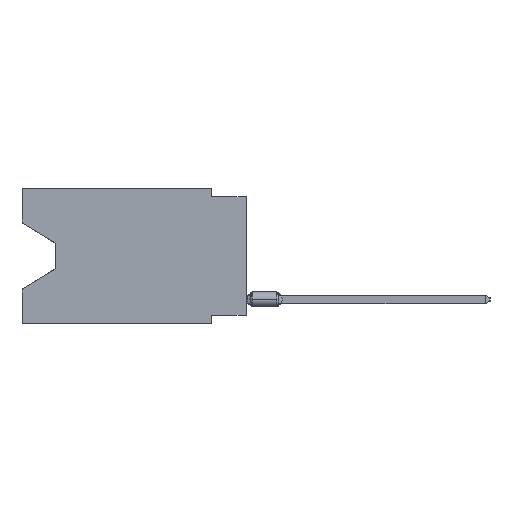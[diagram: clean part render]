
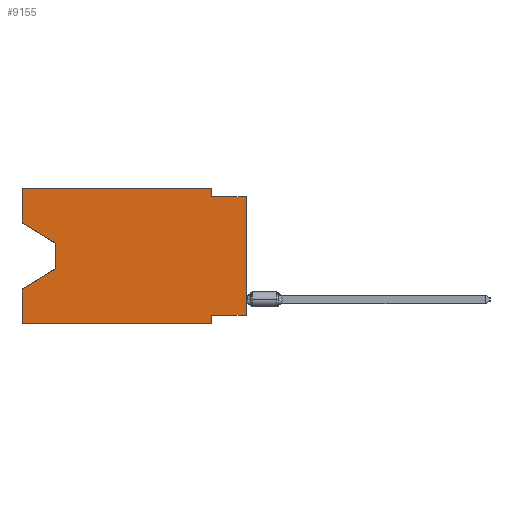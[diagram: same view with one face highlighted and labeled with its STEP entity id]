
A CAD part, left-side view. The second image highlights one B-rep face of the part: STEP entity #9155.
In plain terms, the highlighted planar face has unit normal (-1, 0, 0).
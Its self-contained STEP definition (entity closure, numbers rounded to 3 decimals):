
#777 = CARTESIAN_POINT ( 'NONE',  ( 0., 16.383, -2.546 ) ) ;
#878 = CARTESIAN_POINT ( 'NONE',  ( 0., 16.383, 0. ) ) ;
#1805 = EDGE_CURVE ( 'NONE', #21051, #5855, #35445, .T. ) ;
#2690 = ORIENTED_EDGE ( 'NONE', *, *, #15442, .F. ) ;
#3153 = VERTEX_POINT ( 'NONE', #19789 ) ;
#3461 = VECTOR ( 'NONE', #10659, 1000. ) ;
#3840 = DIRECTION ( 'NONE',  ( 0., 0., -1. ) ) ;
#3842 = VECTOR ( 'NONE', #8933, 1000. ) ;
#4266 = CARTESIAN_POINT ( 'NONE',  ( 0., 16.383, 0. ) ) ;
#4461 = VECTOR ( 'NONE', #26884, 1000. ) ;
#4943 = VERTEX_POINT ( 'NONE', #33859 ) ;
#5568 = ORIENTED_EDGE ( 'NONE', *, *, #12001, .T. ) ;
#5693 = ORIENTED_EDGE ( 'NONE', *, *, #8758, .T. ) ;
#5855 = VERTEX_POINT ( 'NONE', #12146 ) ;
#5992 = ORIENTED_EDGE ( 'NONE', *, *, #22053, .F. ) ;
#6082 = DIRECTION ( 'NONE',  ( 0., 0., 1. ) ) ;
#7894 = CARTESIAN_POINT ( 'NONE',  ( 0., 16.383, 0. ) ) ;
#8083 = CARTESIAN_POINT ( 'NONE',  ( 0., 2.54, -9.906 ) ) ;
#8110 = VECTOR ( 'NONE', #24701, 1000. ) ;
#8553 = LINE ( 'NONE', #17331, #16317 ) ;
#8758 = EDGE_CURVE ( 'NONE', #20627, #10233, #14826, .T. ) ;
#8933 = DIRECTION ( 'NONE',  ( 0., 0., 1. ) ) ;
#9016 = DIRECTION ( 'NONE',  ( 0., -0.855, -0.519 ) ) ;
#9155 = ADVANCED_FACE ( 'NONE', ( #9478 ), #20623, .F. ) ;
#9203 = LINE ( 'NONE', #31097, #34168 ) ;
#9478 = FACE_OUTER_BOUND ( 'NONE', #34843, .T. ) ;
#9645 = DIRECTION ( 'NONE',  ( 0., 0., -1. ) ) ;
#9785 = VECTOR ( 'NONE', #15496, 1000. ) ;
#9920 = LINE ( 'NONE', #34733, #4461 ) ;
#10233 = VERTEX_POINT ( 'NONE', #19840 ) ;
#10643 = DIRECTION ( 'NONE',  ( 0., 0., -1. ) ) ;
#10659 = DIRECTION ( 'NONE',  ( 0., 0., 1. ) ) ;
#10712 = EDGE_CURVE ( 'NONE', #17288, #16648, #11401, .T. ) ;
#11401 = LINE ( 'NONE', #11762, #26263 ) ;
#11762 = CARTESIAN_POINT ( 'NONE',  ( 0., 2.54, 0. ) ) ;
#12001 = EDGE_CURVE ( 'NONE', #21051, #4943, #12758, .T. ) ;
#12146 = CARTESIAN_POINT ( 'NONE',  ( 0., 16.383, -7.36 ) ) ;
#12395 = DIRECTION ( 'NONE',  ( 1., 0., 0. ) ) ;
#12758 = LINE ( 'NONE', #26101, #9785 ) ;
#13210 = CARTESIAN_POINT ( 'NONE',  ( 0., 0., -9.271 ) ) ;
#13745 = ORIENTED_EDGE ( 'NONE', *, *, #15777, .T. ) ;
#14233 = LINE ( 'NONE', #22817, #3842 ) ;
#14826 = LINE ( 'NONE', #18107, #23637 ) ;
#15442 = EDGE_CURVE ( 'NONE', #21552, #22108, #9203, .T. ) ;
#15496 = DIRECTION ( 'NONE',  ( 0., -1., 0. ) ) ;
#15777 = EDGE_CURVE ( 'NONE', #29375, #3153, #14233, .T. ) ;
#16317 = VECTOR ( 'NONE', #25901, 1000. ) ;
#16648 = VERTEX_POINT ( 'NONE', #31653 ) ;
#17288 = VERTEX_POINT ( 'NONE', #33395 ) ;
#17331 = CARTESIAN_POINT ( 'NONE',  ( 0., 13.97, -5.893 ) ) ;
#17620 = EDGE_CURVE ( 'NONE', #21552, #20627, #35683, .T. ) ;
#17624 = AXIS2_PLACEMENT_3D ( 'NONE', #878, #12395, #9645 ) ;
#18068 = VECTOR ( 'NONE', #33264, 1000. ) ;
#18107 = CARTESIAN_POINT ( 'NONE',  ( 0., 13.97, -4.013 ) ) ;
#18858 = LINE ( 'NONE', #8083, #30719 ) ;
#19449 = DIRECTION ( 'NONE',  ( 0., 0., -1. ) ) ;
#19789 = CARTESIAN_POINT ( 'NONE',  ( 0., 0., -0.635 ) ) ;
#19840 = CARTESIAN_POINT ( 'NONE',  ( 0., 13.97, -5.893 ) ) ;
#20623 = PLANE ( 'NONE',  #17624 ) ;
#20627 = VERTEX_POINT ( 'NONE', #34380 ) ;
#21051 = VERTEX_POINT ( 'NONE', #29037 ) ;
#21552 = VERTEX_POINT ( 'NONE', #29484 ) ;
#21555 = CARTESIAN_POINT ( 'NONE',  ( 0., 2.54, -9.271 ) ) ;
#21807 = ORIENTED_EDGE ( 'NONE', *, *, #24415, .F. ) ;
#21870 = EDGE_CURVE ( 'NONE', #29375, #27131, #9920, .T. ) ;
#22053 = EDGE_CURVE ( 'NONE', #27131, #4943, #18858, .T. ) ;
#22108 = VERTEX_POINT ( 'NONE', #7894 ) ;
#22502 = LINE ( 'NONE', #33622, #18068 ) ;
#22519 = LINE ( 'NONE', #35803, #8110 ) ;
#22817 = CARTESIAN_POINT ( 'NONE',  ( 0., 0., 0. ) ) ;
#23637 = VECTOR ( 'NONE', #3840, 1000. ) ;
#24415 = EDGE_CURVE ( 'NONE', #16648, #3153, #22519, .T. ) ;
#24701 = DIRECTION ( 'NONE',  ( 0., -1., 0. ) ) ;
#24954 = ORIENTED_EDGE ( 'NONE', *, *, #21870, .F. ) ;
#25515 = VECTOR ( 'NONE', #9016, 1000. ) ;
#25901 = DIRECTION ( 'NONE',  ( 0., 0.855, -0.519 ) ) ;
#26101 = CARTESIAN_POINT ( 'NONE',  ( 0., 16.383, -9.906 ) ) ;
#26263 = VECTOR ( 'NONE', #19449, 1000. ) ;
#26801 = EDGE_CURVE ( 'NONE', #22108, #17288, #22502, .T. ) ;
#26884 = DIRECTION ( 'NONE',  ( 0., 1., 0. ) ) ;
#27131 = VERTEX_POINT ( 'NONE', #21555 ) ;
#29037 = CARTESIAN_POINT ( 'NONE',  ( 0., 16.383, -9.906 ) ) ;
#29375 = VERTEX_POINT ( 'NONE', #13210 ) ;
#29484 = CARTESIAN_POINT ( 'NONE',  ( 0., 16.383, -2.546 ) ) ;
#30719 = VECTOR ( 'NONE', #10643, 1000. ) ;
#31086 = ORIENTED_EDGE ( 'NONE', *, *, #17620, .T. ) ;
#31097 = CARTESIAN_POINT ( 'NONE',  ( 0., 16.383, 0. ) ) ;
#31653 = CARTESIAN_POINT ( 'NONE',  ( 0., 2.54, -0.635 ) ) ;
#33224 = ORIENTED_EDGE ( 'NONE', *, *, #10712, .F. ) ;
#33264 = DIRECTION ( 'NONE',  ( 0., -1., 0. ) ) ;
#33395 = CARTESIAN_POINT ( 'NONE',  ( 0., 2.54, 0. ) ) ;
#33622 = CARTESIAN_POINT ( 'NONE',  ( 0., 16.383, 0. ) ) ;
#33859 = CARTESIAN_POINT ( 'NONE',  ( 0., 2.54, -9.906 ) ) ;
#34168 = VECTOR ( 'NONE', #6082, 1000. ) ;
#34380 = CARTESIAN_POINT ( 'NONE',  ( 0., 13.97, -4.013 ) ) ;
#34504 = ORIENTED_EDGE ( 'NONE', *, *, #26801, .F. ) ;
#34574 = ORIENTED_EDGE ( 'NONE', *, *, #34838, .T. ) ;
#34733 = CARTESIAN_POINT ( 'NONE',  ( 0., 0., -9.271 ) ) ;
#34838 = EDGE_CURVE ( 'NONE', #10233, #5855, #8553, .T. ) ;
#34843 = EDGE_LOOP ( 'NONE', ( #31086, #5693, #34574, #35603, #5568, #5992, #24954, #13745, #21807, #33224, #34504, #2690 ) ) ;
#35445 = LINE ( 'NONE', #4266, #3461 ) ;
#35603 = ORIENTED_EDGE ( 'NONE', *, *, #1805, .F. ) ;
#35683 = LINE ( 'NONE', #777, #25515 ) ;
#35803 = CARTESIAN_POINT ( 'NONE',  ( 0., 0., -0.635 ) ) ;
